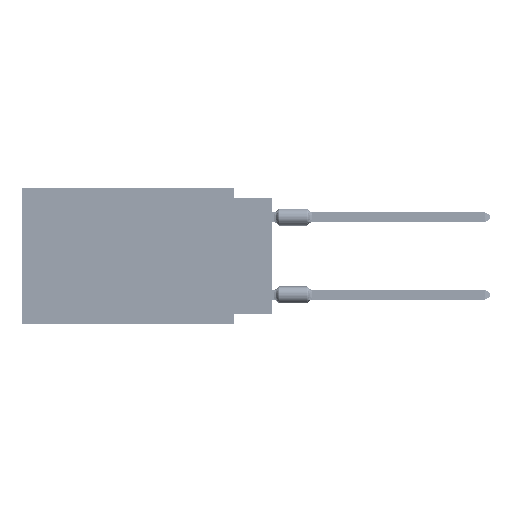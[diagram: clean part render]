
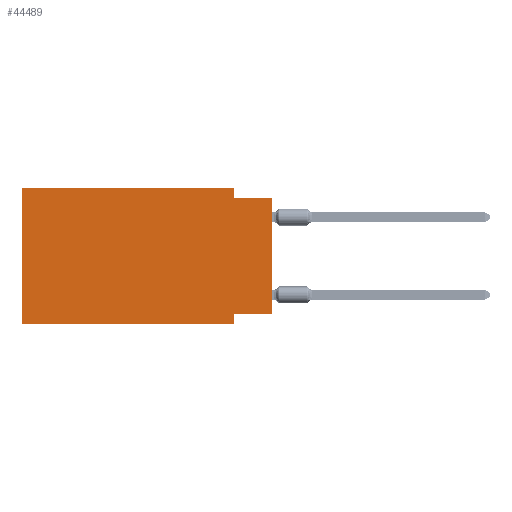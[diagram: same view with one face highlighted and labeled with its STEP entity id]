
A CAD part, left-side view. The second image highlights one B-rep face of the part: STEP entity #44489.
In plain terms, the highlighted planar face has unit normal (-1, 0, 0).
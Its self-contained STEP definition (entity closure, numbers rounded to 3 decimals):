
#609 = CARTESIAN_POINT ( 'NONE',  ( 0., 16.383, -8.89 ) ) ;
#1865 = LINE ( 'NONE', #23897, #63782 ) ;
#2966 = DIRECTION ( 'NONE',  ( 0., 0., -1. ) ) ;
#3037 = VERTEX_POINT ( 'NONE', #17358 ) ;
#3712 = ORIENTED_EDGE ( 'NONE', *, *, #31669, .F. ) ;
#4194 = VECTOR ( 'NONE', #14797, 1000. ) ;
#4314 = LINE ( 'NONE', #46098, #6527 ) ;
#6527 = VECTOR ( 'NONE', #59911, 1000. ) ;
#8174 = VECTOR ( 'NONE', #41503, 1000. ) ;
#10655 = LINE ( 'NONE', #46937, #42460 ) ;
#12454 = VECTOR ( 'NONE', #21782, 1000. ) ;
#13482 = LINE ( 'NONE', #609, #8174 ) ;
#14797 = DIRECTION ( 'NONE',  ( 0., 1., 0. ) ) ;
#15195 = DIRECTION ( 'NONE',  ( 0., 0., 1. ) ) ;
#17358 = CARTESIAN_POINT ( 'NONE',  ( 0., 16.383, 0. ) ) ;
#17578 = VERTEX_POINT ( 'NONE', #20094 ) ;
#20094 = CARTESIAN_POINT ( 'NONE',  ( 0., 2.54, -8.255 ) ) ;
#20276 = ORIENTED_EDGE ( 'NONE', *, *, #89431, .F. ) ;
#21062 = AXIS2_PLACEMENT_3D ( 'NONE', #80126, #79670, #2966 ) ;
#21782 = DIRECTION ( 'NONE',  ( 0., -1., 0. ) ) ;
#22674 = EDGE_LOOP ( 'NONE', ( #50599, #81071, #63699, #48716, #20276, #84165, #3712, #50758 ) ) ;
#23897 = CARTESIAN_POINT ( 'NONE',  ( 0., 0., 0. ) ) ;
#24366 = EDGE_CURVE ( 'NONE', #29425, #83396, #49350, .T. ) ;
#29056 = LINE ( 'NONE', #90631, #4194 ) ;
#29201 = FACE_OUTER_BOUND ( 'NONE', #22674, .T. ) ;
#29425 = VERTEX_POINT ( 'NONE', #30944 ) ;
#30944 = CARTESIAN_POINT ( 'NONE',  ( 0., 2.54, -0.635 ) ) ;
#31669 = EDGE_CURVE ( 'NONE', #17578, #51382, #52184, .T. ) ;
#33158 = DIRECTION ( 'NONE',  ( 0., -1., 0. ) ) ;
#33296 = EDGE_CURVE ( 'NONE', #54666, #29425, #4314, .T. ) ;
#33441 = EDGE_CURVE ( 'NONE', #58857, #83396, #1865, .T. ) ;
#34747 = EDGE_CURVE ( 'NONE', #84248, #51382, #13482, .T. ) ;
#40968 = EDGE_CURVE ( 'NONE', #3037, #54666, #10655, .T. ) ;
#41503 = DIRECTION ( 'NONE',  ( 0., -1., 0. ) ) ;
#42460 = VECTOR ( 'NONE', #33158, 1000. ) ;
#44489 = ADVANCED_FACE ( 'NONE', ( #29201 ), #65450, .F. ) ;
#44587 = CARTESIAN_POINT ( 'NONE',  ( 0., 0., -0.635 ) ) ;
#46098 = CARTESIAN_POINT ( 'NONE',  ( 0., 2.54, 0. ) ) ;
#46937 = CARTESIAN_POINT ( 'NONE',  ( 0., 16.383, 0. ) ) ;
#48716 = ORIENTED_EDGE ( 'NONE', *, *, #40968, .F. ) ;
#49350 = LINE ( 'NONE', #44587, #12454 ) ;
#50599 = ORIENTED_EDGE ( 'NONE', *, *, #33441, .T. ) ;
#50758 = ORIENTED_EDGE ( 'NONE', *, *, #70860, .F. ) ;
#51382 = VERTEX_POINT ( 'NONE', #60022 ) ;
#51725 = DIRECTION ( 'NONE',  ( 0., 0., -1. ) ) ;
#51745 = CARTESIAN_POINT ( 'NONE',  ( 0., 2.54, 0. ) ) ;
#52184 = LINE ( 'NONE', #79738, #57689 ) ;
#54666 = VERTEX_POINT ( 'NONE', #51745 ) ;
#57689 = VECTOR ( 'NONE', #51725, 1000. ) ;
#58857 = VERTEX_POINT ( 'NONE', #72979 ) ;
#59911 = DIRECTION ( 'NONE',  ( 0., 0., -1. ) ) ;
#60022 = CARTESIAN_POINT ( 'NONE',  ( 0., 2.54, -8.89 ) ) ;
#63699 = ORIENTED_EDGE ( 'NONE', *, *, #33296, .F. ) ;
#63782 = VECTOR ( 'NONE', #15195, 1000. ) ;
#65450 = PLANE ( 'NONE',  #21062 ) ;
#70860 = EDGE_CURVE ( 'NONE', #58857, #17578, #29056, .T. ) ;
#72119 = CARTESIAN_POINT ( 'NONE',  ( 0., 16.383, -8.89 ) ) ;
#72979 = CARTESIAN_POINT ( 'NONE',  ( 0., 0., -8.255 ) ) ;
#77248 = LINE ( 'NONE', #83680, #87110 ) ;
#78221 = CARTESIAN_POINT ( 'NONE',  ( 0., 0., -0.635 ) ) ;
#79670 = DIRECTION ( 'NONE',  ( 1., 0., 0. ) ) ;
#79738 = CARTESIAN_POINT ( 'NONE',  ( 0., 2.54, -8.89 ) ) ;
#80126 = CARTESIAN_POINT ( 'NONE',  ( 0., 16.383, 0. ) ) ;
#81071 = ORIENTED_EDGE ( 'NONE', *, *, #24366, .F. ) ;
#83396 = VERTEX_POINT ( 'NONE', #78221 ) ;
#83680 = CARTESIAN_POINT ( 'NONE',  ( 0., 16.383, 0. ) ) ;
#84165 = ORIENTED_EDGE ( 'NONE', *, *, #34747, .T. ) ;
#84248 = VERTEX_POINT ( 'NONE', #72119 ) ;
#87110 = VECTOR ( 'NONE', #90133, 1000. ) ;
#89431 = EDGE_CURVE ( 'NONE', #84248, #3037, #77248, .T. ) ;
#90133 = DIRECTION ( 'NONE',  ( 0., 0., 1. ) ) ;
#90631 = CARTESIAN_POINT ( 'NONE',  ( 0., 0., -8.255 ) ) ;
